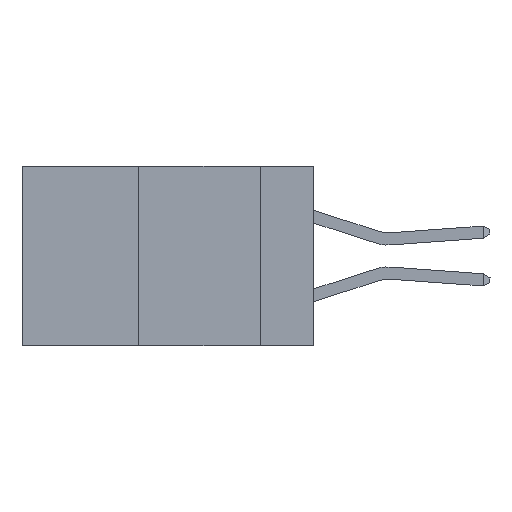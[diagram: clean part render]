
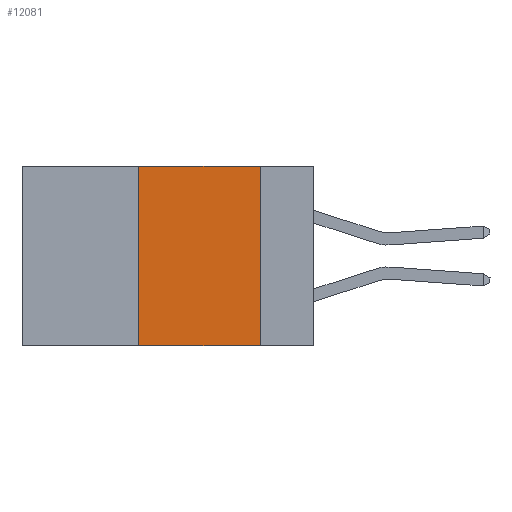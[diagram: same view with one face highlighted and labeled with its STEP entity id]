
A CAD part, left-side view. The second image highlights one B-rep face of the part: STEP entity #12081.
In plain terms, the highlighted planar face has unit normal (-1, 0, 0).
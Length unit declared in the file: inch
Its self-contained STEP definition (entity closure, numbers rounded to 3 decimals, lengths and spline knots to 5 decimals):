
#184 = VERTEX_POINT ( 'NONE', #4241 ) ;
#409 = AXIS2_PLACEMENT_3D ( 'NONE', #1958, #2001, #2875 ) ;
#697 = CARTESIAN_POINT ( 'NONE',  ( 0., 0.6, 0. ) ) ;
#916 = VERTEX_POINT ( 'NONE', #12539 ) ;
#1052 = LINE ( 'NONE', #2216, #3189 ) ;
#1102 = EDGE_LOOP ( 'NONE', ( #11704, #12842, #6433, #8196 ) ) ;
#1260 = VERTEX_POINT ( 'NONE', #7212 ) ;
#1303 = VECTOR ( 'NONE', #12366, 39.37008 ) ;
#1958 = CARTESIAN_POINT ( 'NONE',  ( 0., 0.6, 0. ) ) ;
#2001 = DIRECTION ( 'NONE',  ( 1., 0., 0. ) ) ;
#2216 = CARTESIAN_POINT ( 'NONE',  ( 0., 0.11, 0. ) ) ;
#2423 = LINE ( 'NONE', #3540, #4881 ) ;
#2874 = EDGE_CURVE ( 'NONE', #3358, #916, #1052, .T. ) ;
#2875 = DIRECTION ( 'NONE',  ( 0., 0., -1. ) ) ;
#3189 = VECTOR ( 'NONE', #3241, 39.37008 ) ;
#3241 = DIRECTION ( 'NONE',  ( 0., 0., -1. ) ) ;
#3358 = VERTEX_POINT ( 'NONE', #13682 ) ;
#3540 = CARTESIAN_POINT ( 'NONE',  ( 0., 0.36, 0. ) ) ;
#4045 = EDGE_CURVE ( 'NONE', #1260, #3358, #7434, .T. ) ;
#4241 = CARTESIAN_POINT ( 'NONE',  ( 0., 0.36, -0.37 ) ) ;
#4881 = VECTOR ( 'NONE', #13054, 39.37008 ) ;
#5061 = EDGE_CURVE ( 'NONE', #184, #916, #8368, .T. ) ;
#5631 = VECTOR ( 'NONE', #10141, 39.37008 ) ;
#6433 = ORIENTED_EDGE ( 'NONE', *, *, #10998, .F. ) ;
#7212 = CARTESIAN_POINT ( 'NONE',  ( 0., 0.36, 0. ) ) ;
#7434 = LINE ( 'NONE', #697, #5631 ) ;
#8196 = ORIENTED_EDGE ( 'NONE', *, *, #5061, .T. ) ;
#8368 = LINE ( 'NONE', #10228, #1303 ) ;
#10141 = DIRECTION ( 'NONE',  ( 0., -1., 0. ) ) ;
#10228 = CARTESIAN_POINT ( 'NONE',  ( 0., 0.6, -0.37 ) ) ;
#10998 = EDGE_CURVE ( 'NONE', #184, #1260, #2423, .T. ) ;
#11649 = FACE_OUTER_BOUND ( 'NONE', #1102, .T. ) ;
#11704 = ORIENTED_EDGE ( 'NONE', *, *, #2874, .F. ) ;
#12081 = ADVANCED_FACE ( 'NONE', ( #11649 ), #13467, .F. ) ;
#12366 = DIRECTION ( 'NONE',  ( 0., -1., 0. ) ) ;
#12539 = CARTESIAN_POINT ( 'NONE',  ( 0., 0.11, -0.37 ) ) ;
#12842 = ORIENTED_EDGE ( 'NONE', *, *, #4045, .F. ) ;
#13054 = DIRECTION ( 'NONE',  ( 0., 0., 1. ) ) ;
#13467 = PLANE ( 'NONE',  #409 ) ;
#13682 = CARTESIAN_POINT ( 'NONE',  ( 0., 0.11, 0. ) ) ;
